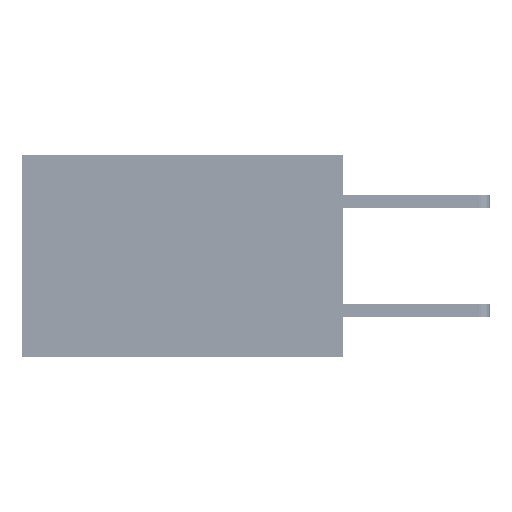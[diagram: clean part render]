
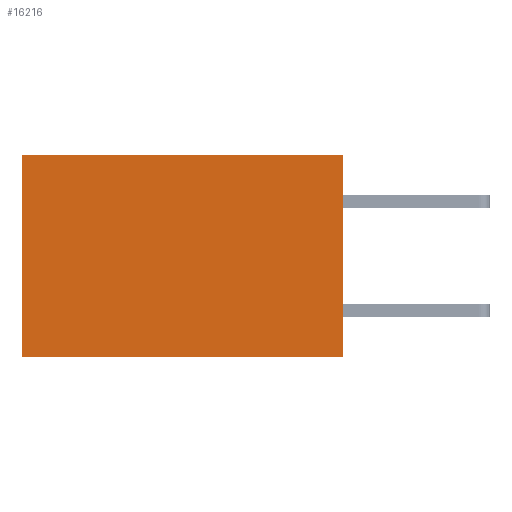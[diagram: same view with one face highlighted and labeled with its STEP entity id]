
A CAD part, left-side view. The second image highlights one B-rep face of the part: STEP entity #16216.
In plain terms, the highlighted planar face has unit normal (-1, 0, 0).
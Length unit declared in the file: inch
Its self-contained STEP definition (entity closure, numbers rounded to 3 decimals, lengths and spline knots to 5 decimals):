
#1590 = VECTOR ( 'NONE', #18033, 39.37008 ) ;
#2179 = CARTESIAN_POINT ( 'NONE',  ( 0.277, 0.59, -0.37 ) ) ;
#2580 = CARTESIAN_POINT ( 'NONE',  ( 0.277, 0., -0.37 ) ) ;
#3070 = VECTOR ( 'NONE', #21975, 39.37008 ) ;
#4544 = VERTEX_POINT ( 'NONE', #2179 ) ;
#5154 = CARTESIAN_POINT ( 'NONE',  ( 0.277, 0.59, 0. ) ) ;
#6285 = CARTESIAN_POINT ( 'NONE',  ( 0.277, 0., -0.37 ) ) ;
#8636 = AXIS2_PLACEMENT_3D ( 'NONE', #27971, #12545, #30521 ) ;
#9447 = CARTESIAN_POINT ( 'NONE',  ( 0.277, 0., 0. ) ) ;
#10031 = ORIENTED_EDGE ( 'NONE', *, *, #11480, .F. ) ;
#10147 = ORIENTED_EDGE ( 'NONE', *, *, #17215, .F. ) ;
#10701 = EDGE_CURVE ( 'NONE', #23018, #4544, #23609, .T. ) ;
#11480 = EDGE_CURVE ( 'NONE', #17329, #13800, #30152, .T. ) ;
#12545 = DIRECTION ( 'NONE',  ( 1., 0., 0. ) ) ;
#13800 = VERTEX_POINT ( 'NONE', #2580 ) ;
#14492 = LINE ( 'NONE', #25764, #1590 ) ;
#16216 = ADVANCED_FACE ( 'NONE', ( #28774 ), #25375, .F. ) ;
#17215 = EDGE_CURVE ( 'NONE', #13800, #4544, #26282, .T. ) ;
#17329 = VERTEX_POINT ( 'NONE', #9447 ) ;
#18033 = DIRECTION ( 'NONE',  ( 0., 1., 0. ) ) ;
#18975 = DIRECTION ( 'NONE',  ( 0., 0., -1. ) ) ;
#19243 = EDGE_CURVE ( 'NONE', #17329, #23018, #14492, .T. ) ;
#19398 = CARTESIAN_POINT ( 'NONE',  ( 0.277, 0.59, -0.37 ) ) ;
#20145 = ORIENTED_EDGE ( 'NONE', *, *, #19243, .T. ) ;
#21455 = CARTESIAN_POINT ( 'NONE',  ( 0.277, 0., -0.37 ) ) ;
#21975 = DIRECTION ( 'NONE',  ( 0., 0., -1. ) ) ;
#22225 = EDGE_LOOP ( 'NONE', ( #28673, #10147, #10031, #20145 ) ) ;
#23018 = VERTEX_POINT ( 'NONE', #5154 ) ;
#23338 = VECTOR ( 'NONE', #18975, 39.37008 ) ;
#23609 = LINE ( 'NONE', #19398, #3070 ) ;
#25375 = PLANE ( 'NONE',  #8636 ) ;
#25764 = CARTESIAN_POINT ( 'NONE',  ( 0.277, 0., 0. ) ) ;
#26282 = LINE ( 'NONE', #6285, #31465 ) ;
#27971 = CARTESIAN_POINT ( 'NONE',  ( 0.277, 0., -0.37 ) ) ;
#28673 = ORIENTED_EDGE ( 'NONE', *, *, #10701, .T. ) ;
#28774 = FACE_OUTER_BOUND ( 'NONE', #22225, .T. ) ;
#30152 = LINE ( 'NONE', #21455, #23338 ) ;
#30521 = DIRECTION ( 'NONE',  ( 0., 0., -1. ) ) ;
#31465 = VECTOR ( 'NONE', #32029, 39.37008 ) ;
#32029 = DIRECTION ( 'NONE',  ( 0., 1., 0. ) ) ;
